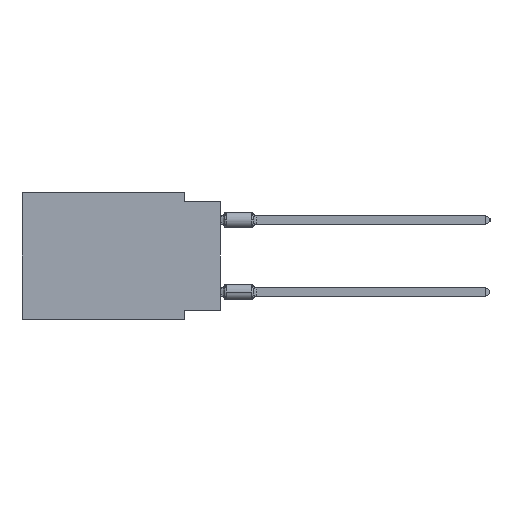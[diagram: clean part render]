
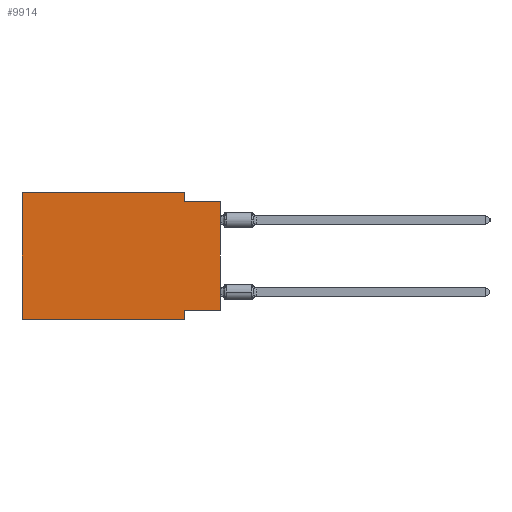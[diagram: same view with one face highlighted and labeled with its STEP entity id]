
A CAD part, left-side view. The second image highlights one B-rep face of the part: STEP entity #9914.
In plain terms, the highlighted planar face has unit normal (-1, 0, 0).
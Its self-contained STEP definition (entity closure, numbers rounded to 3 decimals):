
#104 = EDGE_LOOP ( 'NONE', ( #3951, #15416, #26189, #4099, #13747, #32416, #23814, #10241 ) ) ;
#1587 = DIRECTION ( 'NONE',  ( 0., 0., -1. ) ) ;
#1741 = PLANE ( 'NONE',  #10619 ) ;
#3400 = EDGE_CURVE ( 'NONE', #14539, #23685, #29160, .T. ) ;
#3570 = VERTEX_POINT ( 'NONE', #20478 ) ;
#3951 = ORIENTED_EDGE ( 'NONE', *, *, #22051, .T. ) ;
#4099 = ORIENTED_EDGE ( 'NONE', *, *, #27119, .F. ) ;
#6573 = CARTESIAN_POINT ( 'NONE',  ( 0., 0., 0. ) ) ;
#7894 = EDGE_CURVE ( 'NONE', #18489, #32250, #14521, .T. ) ;
#8033 = CARTESIAN_POINT ( 'NONE',  ( 0., 13.97, 0. ) ) ;
#8262 = CARTESIAN_POINT ( 'NONE',  ( 0., 2.54, -8.89 ) ) ;
#9331 = CARTESIAN_POINT ( 'NONE',  ( 0., 2.54, 0. ) ) ;
#9914 = ADVANCED_FACE ( 'NONE', ( #12629 ), #1741, .F. ) ;
#10061 = CARTESIAN_POINT ( 'NONE',  ( 0., 2.54, -8.255 ) ) ;
#10241 = ORIENTED_EDGE ( 'NONE', *, *, #7894, .F. ) ;
#10619 = AXIS2_PLACEMENT_3D ( 'NONE', #20230, #23143, #1587 ) ;
#10781 = VECTOR ( 'NONE', #14018, 1000. ) ;
#10865 = DIRECTION ( 'NONE',  ( 0., -1., 0. ) ) ;
#11063 = CARTESIAN_POINT ( 'NONE',  ( 0., 2.54, 0. ) ) ;
#12629 = FACE_OUTER_BOUND ( 'NONE', #104, .T. ) ;
#12652 = EDGE_CURVE ( 'NONE', #32250, #23685, #26887, .T. ) ;
#12986 = VECTOR ( 'NONE', #14843, 1000. ) ;
#13747 = ORIENTED_EDGE ( 'NONE', *, *, #23162, .F. ) ;
#14018 = DIRECTION ( 'NONE',  ( 0., 1., 0. ) ) ;
#14521 = LINE ( 'NONE', #16956, #10781 ) ;
#14539 = VERTEX_POINT ( 'NONE', #26532 ) ;
#14695 = LINE ( 'NONE', #6573, #16120 ) ;
#14843 = DIRECTION ( 'NONE',  ( 0., 0., -1. ) ) ;
#15416 = ORIENTED_EDGE ( 'NONE', *, *, #22974, .F. ) ;
#16120 = VECTOR ( 'NONE', #17268, 1000. ) ;
#16956 = CARTESIAN_POINT ( 'NONE',  ( 0., 0., -8.255 ) ) ;
#17268 = DIRECTION ( 'NONE',  ( 0., 0., 1. ) ) ;
#18489 = VERTEX_POINT ( 'NONE', #19773 ) ;
#18547 = LINE ( 'NONE', #26970, #33235 ) ;
#18564 = DIRECTION ( 'NONE',  ( 0., -1., 0. ) ) ;
#18850 = DIRECTION ( 'NONE',  ( 0., 0., 1. ) ) ;
#18933 = VECTOR ( 'NONE', #28705, 1000. ) ;
#19773 = CARTESIAN_POINT ( 'NONE',  ( 0., 0., -8.255 ) ) ;
#20230 = CARTESIAN_POINT ( 'NONE',  ( 0., 13.97, 0. ) ) ;
#20411 = EDGE_CURVE ( 'NONE', #21331, #26957, #20520, .T. ) ;
#20478 = CARTESIAN_POINT ( 'NONE',  ( 0., 0., -0.635 ) ) ;
#20520 = LINE ( 'NONE', #9331, #12986 ) ;
#21331 = VERTEX_POINT ( 'NONE', #11063 ) ;
#21853 = VECTOR ( 'NONE', #10865, 1000. ) ;
#22051 = EDGE_CURVE ( 'NONE', #18489, #3570, #14695, .T. ) ;
#22938 = CARTESIAN_POINT ( 'NONE',  ( 0., 2.54, -8.89 ) ) ;
#22974 = EDGE_CURVE ( 'NONE', #26957, #3570, #28363, .T. ) ;
#23143 = DIRECTION ( 'NONE',  ( 1., 0., 0. ) ) ;
#23162 = EDGE_CURVE ( 'NONE', #14539, #27957, #18547, .T. ) ;
#23685 = VERTEX_POINT ( 'NONE', #22938 ) ;
#23715 = LINE ( 'NONE', #8033, #30596 ) ;
#23814 = ORIENTED_EDGE ( 'NONE', *, *, #12652, .F. ) ;
#24981 = VECTOR ( 'NONE', #29637, 1000. ) ;
#26065 = CARTESIAN_POINT ( 'NONE',  ( 0., 13.97, 0. ) ) ;
#26189 = ORIENTED_EDGE ( 'NONE', *, *, #20411, .F. ) ;
#26532 = CARTESIAN_POINT ( 'NONE',  ( 0., 13.97, -8.89 ) ) ;
#26550 = CARTESIAN_POINT ( 'NONE',  ( 0., 13.97, -8.89 ) ) ;
#26887 = LINE ( 'NONE', #8262, #24981 ) ;
#26957 = VERTEX_POINT ( 'NONE', #27869 ) ;
#26970 = CARTESIAN_POINT ( 'NONE',  ( 0., 13.97, 0. ) ) ;
#27119 = EDGE_CURVE ( 'NONE', #27957, #21331, #23715, .T. ) ;
#27869 = CARTESIAN_POINT ( 'NONE',  ( 0., 2.54, -0.635 ) ) ;
#27957 = VERTEX_POINT ( 'NONE', #26065 ) ;
#28363 = LINE ( 'NONE', #33547, #18933 ) ;
#28705 = DIRECTION ( 'NONE',  ( 0., -1., 0. ) ) ;
#29160 = LINE ( 'NONE', #26550, #21853 ) ;
#29637 = DIRECTION ( 'NONE',  ( 0., 0., -1. ) ) ;
#30596 = VECTOR ( 'NONE', #18564, 1000. ) ;
#32250 = VERTEX_POINT ( 'NONE', #10061 ) ;
#32416 = ORIENTED_EDGE ( 'NONE', *, *, #3400, .T. ) ;
#33235 = VECTOR ( 'NONE', #18850, 1000. ) ;
#33547 = CARTESIAN_POINT ( 'NONE',  ( 0., 0., -0.635 ) ) ;
